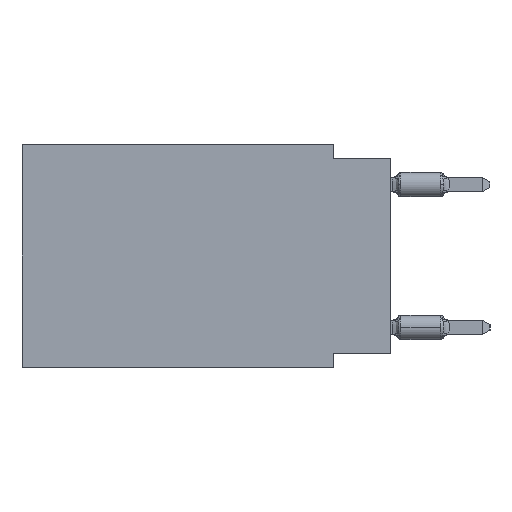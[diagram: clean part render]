
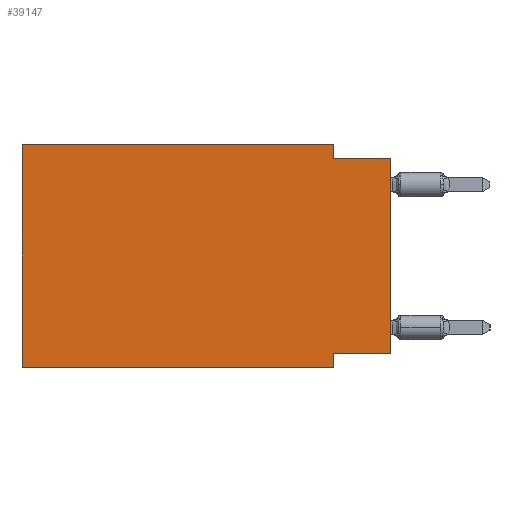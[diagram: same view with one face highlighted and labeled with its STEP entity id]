
A CAD part, left-side view. The second image highlights one B-rep face of the part: STEP entity #39147.
In plain terms, the highlighted planar face has unit normal (-1, 0, 0).
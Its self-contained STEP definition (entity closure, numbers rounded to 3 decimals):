
#1111 = DIRECTION ( 'NONE',  ( 0., 0., -1. ) ) ;
#2074 = PLANE ( 'NONE',  #32900 ) ;
#2442 = DIRECTION ( 'NONE',  ( 0., 0., 1. ) ) ;
#2990 = ORIENTED_EDGE ( 'NONE', *, *, #56008, .F. ) ;
#4312 = DIRECTION ( 'NONE',  ( 0., -1., 0. ) ) ;
#4404 = VERTEX_POINT ( 'NONE', #62261 ) ;
#4870 = CARTESIAN_POINT ( 'NONE',  ( 0., 0., -0.635 ) ) ;
#5360 = VECTOR ( 'NONE', #19596, 1000. ) ;
#7233 = CARTESIAN_POINT ( 'NONE',  ( 0., 16.383, 0. ) ) ;
#8465 = DIRECTION ( 'NONE',  ( 0., -1., 0. ) ) ;
#10498 = ORIENTED_EDGE ( 'NONE', *, *, #48890, .F. ) ;
#11132 = VECTOR ( 'NONE', #2442, 1000. ) ;
#11456 = VECTOR ( 'NONE', #18615, 1000. ) ;
#11831 = EDGE_CURVE ( 'NONE', #45964, #34021, #37913, .T. ) ;
#11855 = DIRECTION ( 'NONE',  ( 0., 1., 0. ) ) ;
#12003 = DIRECTION ( 'NONE',  ( 1., 0., 0. ) ) ;
#12495 = LINE ( 'NONE', #45867, #25972 ) ;
#12690 = CARTESIAN_POINT ( 'NONE',  ( 0., 0., -9.271 ) ) ;
#13138 = EDGE_CURVE ( 'NONE', #17849, #4404, #24728, .T. ) ;
#14164 = ORIENTED_EDGE ( 'NONE', *, *, #13138, .F. ) ;
#17680 = ORIENTED_EDGE ( 'NONE', *, *, #61800, .F. ) ;
#17849 = VERTEX_POINT ( 'NONE', #30092 ) ;
#18534 = VERTEX_POINT ( 'NONE', #29867 ) ;
#18615 = DIRECTION ( 'NONE',  ( 0., 0., -1. ) ) ;
#19596 = DIRECTION ( 'NONE',  ( 0., -1., 0. ) ) ;
#19906 = LINE ( 'NONE', #58423, #5360 ) ;
#24073 = ORIENTED_EDGE ( 'NONE', *, *, #11831, .T. ) ;
#24728 = LINE ( 'NONE', #34053, #39658 ) ;
#25475 = FACE_OUTER_BOUND ( 'NONE', #33222, .T. ) ;
#25972 = VECTOR ( 'NONE', #11855, 1000. ) ;
#28275 = VECTOR ( 'NONE', #8465, 1000. ) ;
#28677 = CARTESIAN_POINT ( 'NONE',  ( 0., 16.383, -9.906 ) ) ;
#29867 = CARTESIAN_POINT ( 'NONE',  ( 0., 16.383, -9.906 ) ) ;
#29894 = VERTEX_POINT ( 'NONE', #56967 ) ;
#30092 = CARTESIAN_POINT ( 'NONE',  ( 0., 2.54, -9.271 ) ) ;
#32900 = AXIS2_PLACEMENT_3D ( 'NONE', #45067, #12003, #1111 ) ;
#33222 = EDGE_LOOP ( 'NONE', ( #24073, #10498, #17680, #2990, #41131, #41347, #14164, #34907 ) ) ;
#33411 = DIRECTION ( 'NONE',  ( 0., 0., 1. ) ) ;
#34021 = VERTEX_POINT ( 'NONE', #4870 ) ;
#34053 = CARTESIAN_POINT ( 'NONE',  ( 0., 2.54, -9.906 ) ) ;
#34907 = ORIENTED_EDGE ( 'NONE', *, *, #42738, .F. ) ;
#35081 = VERTEX_POINT ( 'NONE', #39160 ) ;
#35941 = EDGE_CURVE ( 'NONE', #18534, #4404, #59135, .T. ) ;
#37871 = CARTESIAN_POINT ( 'NONE',  ( 0., 2.54, 0. ) ) ;
#37913 = LINE ( 'NONE', #38231, #47742 ) ;
#38231 = CARTESIAN_POINT ( 'NONE',  ( 0., 0., 0. ) ) ;
#39147 = ADVANCED_FACE ( 'NONE', ( #25475 ), #2074, .F. ) ;
#39160 = CARTESIAN_POINT ( 'NONE',  ( 0., 2.54, 0. ) ) ;
#39658 = VECTOR ( 'NONE', #59705, 1000. ) ;
#41131 = ORIENTED_EDGE ( 'NONE', *, *, #58295, .F. ) ;
#41347 = ORIENTED_EDGE ( 'NONE', *, *, #35941, .T. ) ;
#42738 = EDGE_CURVE ( 'NONE', #45964, #17849, #12495, .T. ) ;
#42847 = VECTOR ( 'NONE', #4312, 1000. ) ;
#45067 = CARTESIAN_POINT ( 'NONE',  ( 0., 16.383, 0. ) ) ;
#45867 = CARTESIAN_POINT ( 'NONE',  ( 0., 0., -9.271 ) ) ;
#45964 = VERTEX_POINT ( 'NONE', #12690 ) ;
#47742 = VECTOR ( 'NONE', #33411, 1000. ) ;
#48239 = LINE ( 'NONE', #52430, #28275 ) ;
#48890 = EDGE_CURVE ( 'NONE', #29894, #34021, #48239, .T. ) ;
#51504 = LINE ( 'NONE', #7233, #11132 ) ;
#52430 = CARTESIAN_POINT ( 'NONE',  ( 0., 0., -0.635 ) ) ;
#54810 = VERTEX_POINT ( 'NONE', #58720 ) ;
#56008 = EDGE_CURVE ( 'NONE', #54810, #35081, #19906, .T. ) ;
#56967 = CARTESIAN_POINT ( 'NONE',  ( 0., 2.54, -0.635 ) ) ;
#57445 = LINE ( 'NONE', #37871, #11456 ) ;
#58295 = EDGE_CURVE ( 'NONE', #18534, #54810, #51504, .T. ) ;
#58423 = CARTESIAN_POINT ( 'NONE',  ( 0., 16.383, 0. ) ) ;
#58720 = CARTESIAN_POINT ( 'NONE',  ( 0., 16.383, 0. ) ) ;
#59135 = LINE ( 'NONE', #28677, #42847 ) ;
#59705 = DIRECTION ( 'NONE',  ( 0., 0., -1. ) ) ;
#61800 = EDGE_CURVE ( 'NONE', #35081, #29894, #57445, .T. ) ;
#62261 = CARTESIAN_POINT ( 'NONE',  ( 0., 2.54, -9.906 ) ) ;
